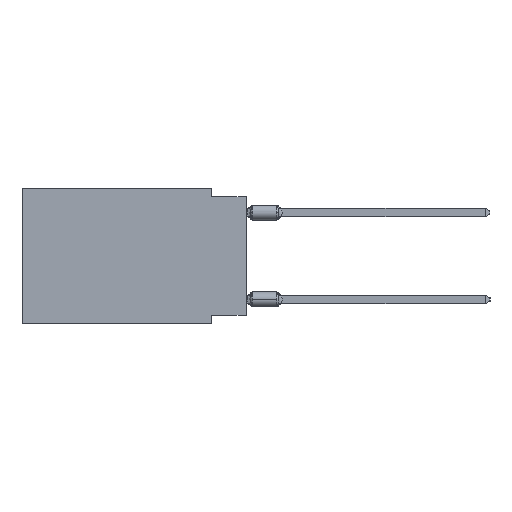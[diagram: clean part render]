
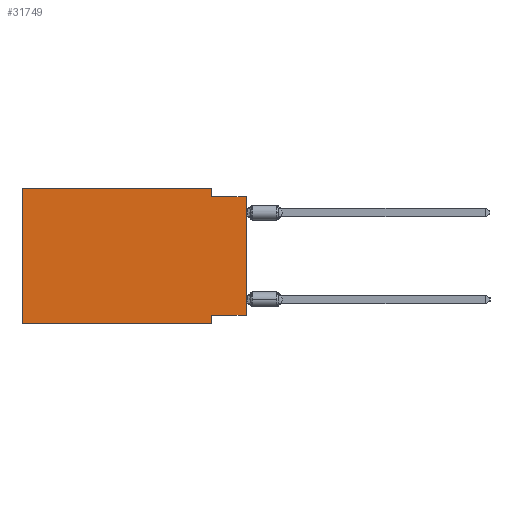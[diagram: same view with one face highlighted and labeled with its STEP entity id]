
A CAD part, left-side view. The second image highlights one B-rep face of the part: STEP entity #31749.
In plain terms, the highlighted planar face has unit normal (-1, 0, 0).
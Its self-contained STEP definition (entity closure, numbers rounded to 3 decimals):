
#2041 = CARTESIAN_POINT ( 'NONE',  ( 0., 16.383, -9.906 ) ) ;
#3770 = ORIENTED_EDGE ( 'NONE', *, *, #6444, .F. ) ;
#3946 = EDGE_CURVE ( 'NONE', #35198, #30519, #22612, .T. ) ;
#6444 = EDGE_CURVE ( 'NONE', #41694, #35198, #27269, .T. ) ;
#6833 = LINE ( 'NONE', #7048, #43417 ) ;
#7048 = CARTESIAN_POINT ( 'NONE',  ( 0., 16.383, 0. ) ) ;
#7271 = DIRECTION ( 'NONE',  ( 0., 1., 0. ) ) ;
#7334 = LINE ( 'NONE', #30192, #32045 ) ;
#7571 = VERTEX_POINT ( 'NONE', #29559 ) ;
#9846 = VERTEX_POINT ( 'NONE', #32423 ) ;
#11300 = DIRECTION ( 'NONE',  ( 0., 0., -1. ) ) ;
#11310 = DIRECTION ( 'NONE',  ( 0., 0., -1. ) ) ;
#11664 = ORIENTED_EDGE ( 'NONE', *, *, #18986, .F. ) ;
#12410 = ORIENTED_EDGE ( 'NONE', *, *, #30459, .F. ) ;
#12612 = EDGE_CURVE ( 'NONE', #30381, #20925, #7334, .T. ) ;
#12840 = EDGE_LOOP ( 'NONE', ( #40251, #43802, #3770, #12410, #11664, #15132, #31679, #37474 ) ) ;
#13467 = CARTESIAN_POINT ( 'NONE',  ( 0., 16.383, 0. ) ) ;
#14606 = CARTESIAN_POINT ( 'NONE',  ( 0., 2.54, -0.635 ) ) ;
#15132 = ORIENTED_EDGE ( 'NONE', *, *, #18374, .T. ) ;
#15144 = VECTOR ( 'NONE', #11310, 1000. ) ;
#15186 = VERTEX_POINT ( 'NONE', #33535 ) ;
#15586 = DIRECTION ( 'NONE',  ( 1., 0., 0. ) ) ;
#15628 = EDGE_CURVE ( 'NONE', #15186, #30519, #19244, .T. ) ;
#17946 = CARTESIAN_POINT ( 'NONE',  ( 0., 2.54, -9.906 ) ) ;
#18374 = EDGE_CURVE ( 'NONE', #7571, #20925, #28390, .T. ) ;
#18720 = PLANE ( 'NONE',  #32148 ) ;
#18986 = EDGE_CURVE ( 'NONE', #7571, #9846, #30095, .T. ) ;
#19244 = LINE ( 'NONE', #42099, #41321 ) ;
#19859 = VECTOR ( 'NONE', #37393, 1000. ) ;
#20925 = VERTEX_POINT ( 'NONE', #17946 ) ;
#21268 = DIRECTION ( 'NONE',  ( 0., -1., 0. ) ) ;
#22357 = DIRECTION ( 'NONE',  ( 0., 0., 1. ) ) ;
#22612 = LINE ( 'NONE', #31007, #40279 ) ;
#26552 = DIRECTION ( 'NONE',  ( 0., -1., 0. ) ) ;
#27269 = LINE ( 'NONE', #41009, #15144 ) ;
#27430 = LINE ( 'NONE', #37607, #33191 ) ;
#28390 = LINE ( 'NONE', #2041, #40347 ) ;
#29559 = CARTESIAN_POINT ( 'NONE',  ( 0., 16.383, -9.906 ) ) ;
#29981 = DIRECTION ( 'NONE',  ( 0., 0., -1. ) ) ;
#30095 = LINE ( 'NONE', #13467, #19859 ) ;
#30192 = CARTESIAN_POINT ( 'NONE',  ( 0., 2.54, -9.906 ) ) ;
#30381 = VERTEX_POINT ( 'NONE', #42371 ) ;
#30459 = EDGE_CURVE ( 'NONE', #9846, #41694, #6833, .T. ) ;
#30519 = VERTEX_POINT ( 'NONE', #43632 ) ;
#31007 = CARTESIAN_POINT ( 'NONE',  ( 0., 0., -0.635 ) ) ;
#31679 = ORIENTED_EDGE ( 'NONE', *, *, #12612, .F. ) ;
#31749 = ADVANCED_FACE ( 'NONE', ( #35320 ), #18720, .F. ) ;
#32045 = VECTOR ( 'NONE', #11300, 1000. ) ;
#32148 = AXIS2_PLACEMENT_3D ( 'NONE', #32205, #15586, #29981 ) ;
#32205 = CARTESIAN_POINT ( 'NONE',  ( 0., 16.383, 0. ) ) ;
#32423 = CARTESIAN_POINT ( 'NONE',  ( 0., 16.383, 0. ) ) ;
#33191 = VECTOR ( 'NONE', #7271, 1000. ) ;
#33535 = CARTESIAN_POINT ( 'NONE',  ( 0., 0., -9.271 ) ) ;
#35198 = VERTEX_POINT ( 'NONE', #14606 ) ;
#35320 = FACE_OUTER_BOUND ( 'NONE', #12840, .T. ) ;
#37393 = DIRECTION ( 'NONE',  ( 0., 0., 1. ) ) ;
#37474 = ORIENTED_EDGE ( 'NONE', *, *, #41941, .F. ) ;
#37607 = CARTESIAN_POINT ( 'NONE',  ( 0., 0., -9.271 ) ) ;
#40251 = ORIENTED_EDGE ( 'NONE', *, *, #15628, .T. ) ;
#40279 = VECTOR ( 'NONE', #21268, 1000. ) ;
#40347 = VECTOR ( 'NONE', #41927, 1000. ) ;
#40825 = CARTESIAN_POINT ( 'NONE',  ( 0., 2.54, 0. ) ) ;
#41009 = CARTESIAN_POINT ( 'NONE',  ( 0., 2.54, 0. ) ) ;
#41321 = VECTOR ( 'NONE', #22357, 1000. ) ;
#41694 = VERTEX_POINT ( 'NONE', #40825 ) ;
#41927 = DIRECTION ( 'NONE',  ( 0., -1., 0. ) ) ;
#41941 = EDGE_CURVE ( 'NONE', #15186, #30381, #27430, .T. ) ;
#42099 = CARTESIAN_POINT ( 'NONE',  ( 0., 0., 0. ) ) ;
#42371 = CARTESIAN_POINT ( 'NONE',  ( 0., 2.54, -9.271 ) ) ;
#43417 = VECTOR ( 'NONE', #26552, 1000. ) ;
#43632 = CARTESIAN_POINT ( 'NONE',  ( 0., 0., -0.635 ) ) ;
#43802 = ORIENTED_EDGE ( 'NONE', *, *, #3946, .F. ) ;
